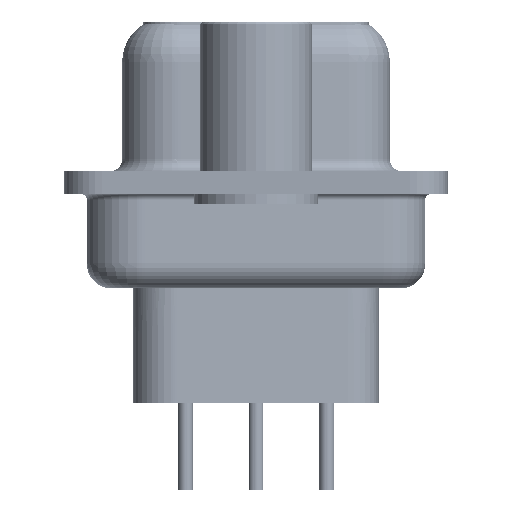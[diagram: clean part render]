
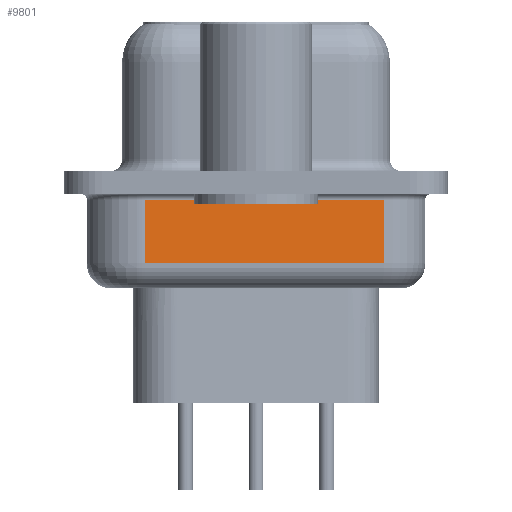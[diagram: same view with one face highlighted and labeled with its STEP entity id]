
A CAD part, left-side view. The second image highlights one B-rep face of the part: STEP entity #9801.
In plain terms, the highlighted planar face has unit normal (-0.985, -0.174, 0).
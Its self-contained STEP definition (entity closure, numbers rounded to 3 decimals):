
#1876 = EDGE_CURVE ( 'NONE', #41035, #13428, #4110, .T. ) ;
#2502 = CARTESIAN_POINT ( 'NONE',  ( 4.623, -5.147, -0.7 ) ) ;
#4110 = LINE ( 'NONE', #4344, #13652 ) ;
#4344 = CARTESIAN_POINT ( 'NONE',  ( 2.93, 4.453, -3.25 ) ) ;
#6392 = CARTESIAN_POINT ( 'NONE',  ( 2.93, 4.453, -4.25 ) ) ;
#9142 = VERTEX_POINT ( 'NONE', #35101 ) ;
#9801 = ADVANCED_FACE ( 'NONE', ( #34222 ), #40720, .F. ) ;
#9968 = LINE ( 'NONE', #6392, #28933 ) ;
#11658 = AXIS2_PLACEMENT_3D ( 'NONE', #12542, #33529, #12305 ) ;
#12305 = DIRECTION ( 'NONE',  ( -0.174, 0.985, 0. ) ) ;
#12542 = CARTESIAN_POINT ( 'NONE',  ( 2.93, 4.453, -4.25 ) ) ;
#13428 = VERTEX_POINT ( 'NONE', #34264 ) ;
#13652 = VECTOR ( 'NONE', #18688, 1000. ) ;
#13927 = CARTESIAN_POINT ( 'NONE',  ( 4.623, -5.147, -4.25 ) ) ;
#14008 = VERTEX_POINT ( 'NONE', #2502 ) ;
#18688 = DIRECTION ( 'NONE',  ( 0.174, -0.985, 0. ) ) ;
#20306 = CARTESIAN_POINT ( 'NONE',  ( 2.93, 4.453, -3.25 ) ) ;
#22719 = EDGE_LOOP ( 'NONE', ( #23171, #31556, #29220, #40872 ) ) ;
#23171 = ORIENTED_EDGE ( 'NONE', *, *, #26130, .F. ) ;
#24406 = DIRECTION ( 'NONE',  ( 0., 0., 1. ) ) ;
#25692 = EDGE_CURVE ( 'NONE', #13428, #14008, #28451, .T. ) ;
#26130 = EDGE_CURVE ( 'NONE', #41035, #9142, #9968, .T. ) ;
#27357 = EDGE_CURVE ( 'NONE', #14008, #9142, #38679, .T. ) ;
#28451 = LINE ( 'NONE', #13927, #37281 ) ;
#28933 = VECTOR ( 'NONE', #45803, 1000. ) ;
#29220 = ORIENTED_EDGE ( 'NONE', *, *, #25692, .T. ) ;
#30557 = DIRECTION ( 'NONE',  ( -0.174, 0.985, 0. ) ) ;
#31556 = ORIENTED_EDGE ( 'NONE', *, *, #1876, .T. ) ;
#33529 = DIRECTION ( 'NONE',  ( 0.985, 0.174, 0. ) ) ;
#34222 = FACE_OUTER_BOUND ( 'NONE', #22719, .T. ) ;
#34264 = CARTESIAN_POINT ( 'NONE',  ( 4.623, -5.147, -3.25 ) ) ;
#35101 = CARTESIAN_POINT ( 'NONE',  ( 2.93, 4.453, -0.7 ) ) ;
#37281 = VECTOR ( 'NONE', #24406, 1000. ) ;
#38679 = LINE ( 'NONE', #42276, #45868 ) ;
#40720 = PLANE ( 'NONE',  #11658 ) ;
#40872 = ORIENTED_EDGE ( 'NONE', *, *, #27357, .T. ) ;
#41035 = VERTEX_POINT ( 'NONE', #20306 ) ;
#42276 = CARTESIAN_POINT ( 'NONE',  ( 2.93, 4.453, -0.7 ) ) ;
#45803 = DIRECTION ( 'NONE',  ( 0., 0., 1. ) ) ;
#45868 = VECTOR ( 'NONE', #30557, 1000. ) ;
